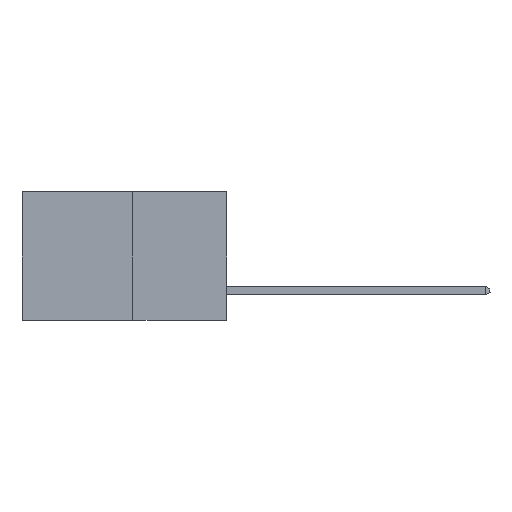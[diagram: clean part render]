
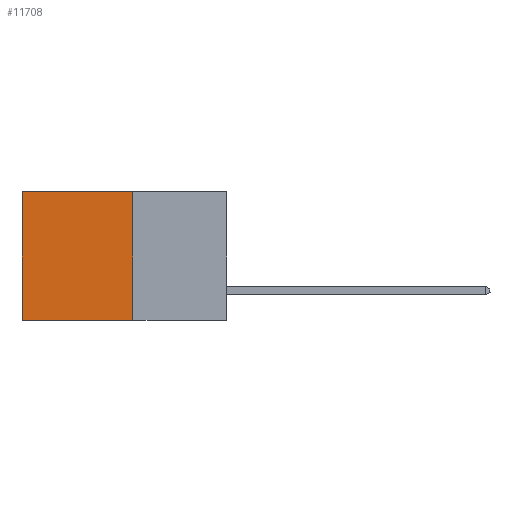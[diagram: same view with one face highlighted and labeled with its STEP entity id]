
A CAD part, left-side view. The second image highlights one B-rep face of the part: STEP entity #11708.
In plain terms, the highlighted planar face has unit normal (-1, 0, 0).
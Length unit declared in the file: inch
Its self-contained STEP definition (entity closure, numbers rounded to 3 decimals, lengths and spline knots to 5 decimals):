
#163 = LINE ( 'NONE', #12467, #4184 ) ;
#827 = VERTEX_POINT ( 'NONE', #14839 ) ;
#1203 = ORIENTED_EDGE ( 'NONE', *, *, #8053, .F. ) ;
#1705 = CARTESIAN_POINT ( 'NONE',  ( 0.277, 0.27, -0.37 ) ) ;
#2343 = DIRECTION ( 'NONE',  ( 0., 0., -1. ) ) ;
#3374 = CARTESIAN_POINT ( 'NONE',  ( 0.277, 0.27, 0. ) ) ;
#4184 = VECTOR ( 'NONE', #2343, 39.37008 ) ;
#5153 = DIRECTION ( 'NONE',  ( 0., 0., -1. ) ) ;
#5385 = ORIENTED_EDGE ( 'NONE', *, *, #7468, .T. ) ;
#5523 = LINE ( 'NONE', #1705, #9010 ) ;
#5834 = VERTEX_POINT ( 'NONE', #18455 ) ;
#6041 = CARTESIAN_POINT ( 'NONE',  ( 0.277, 0.27, 0. ) ) ;
#6504 = AXIS2_PLACEMENT_3D ( 'NONE', #14618, #9690, #21035 ) ;
#6609 = VECTOR ( 'NONE', #14465, 39.37008 ) ;
#7468 = EDGE_CURVE ( 'NONE', #17783, #827, #11121, .T. ) ;
#8053 = EDGE_CURVE ( 'NONE', #14174, #5834, #13439, .T. ) ;
#8307 = FACE_OUTER_BOUND ( 'NONE', #8583, .T. ) ;
#8583 = EDGE_LOOP ( 'NONE', ( #13124, #1203, #20844, #5385 ) ) ;
#8710 = EDGE_CURVE ( 'NONE', #827, #5834, #163, .T. ) ;
#8760 = CARTESIAN_POINT ( 'NONE',  ( 0.277, 0.27, -0.37 ) ) ;
#9010 = VECTOR ( 'NONE', #5153, 39.37008 ) ;
#9690 = DIRECTION ( 'NONE',  ( 1., 0., 0. ) ) ;
#11121 = LINE ( 'NONE', #6041, #6609 ) ;
#11708 = ADVANCED_FACE ( 'NONE', ( #8307 ), #19438, .F. ) ;
#12467 = CARTESIAN_POINT ( 'NONE',  ( 0.277, 0.59, -0.37 ) ) ;
#12902 = VECTOR ( 'NONE', #15770, 39.37008 ) ;
#13124 = ORIENTED_EDGE ( 'NONE', *, *, #8710, .T. ) ;
#13439 = LINE ( 'NONE', #14162, #12902 ) ;
#14162 = CARTESIAN_POINT ( 'NONE',  ( 0.277, 0.27, -0.37 ) ) ;
#14174 = VERTEX_POINT ( 'NONE', #8760 ) ;
#14465 = DIRECTION ( 'NONE',  ( 0., 1., 0. ) ) ;
#14618 = CARTESIAN_POINT ( 'NONE',  ( 0.277, 0.27, -0.37 ) ) ;
#14639 = EDGE_CURVE ( 'NONE', #17783, #14174, #5523, .T. ) ;
#14839 = CARTESIAN_POINT ( 'NONE',  ( 0.277, 0.59, 0. ) ) ;
#15770 = DIRECTION ( 'NONE',  ( 0., 1., 0. ) ) ;
#17783 = VERTEX_POINT ( 'NONE', #3374 ) ;
#18455 = CARTESIAN_POINT ( 'NONE',  ( 0.277, 0.59, -0.37 ) ) ;
#19438 = PLANE ( 'NONE',  #6504 ) ;
#20844 = ORIENTED_EDGE ( 'NONE', *, *, #14639, .F. ) ;
#21035 = DIRECTION ( 'NONE',  ( 0., 0., -1. ) ) ;
